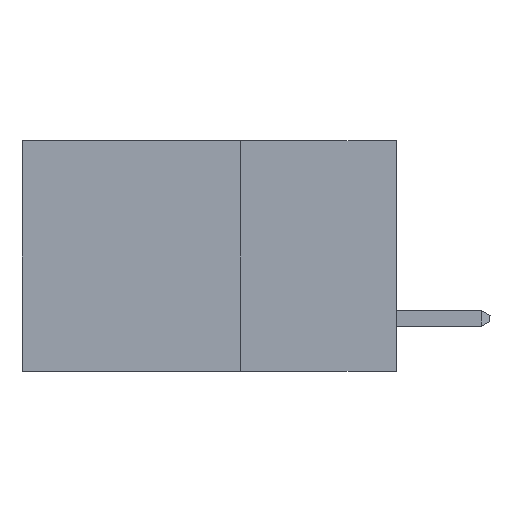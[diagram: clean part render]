
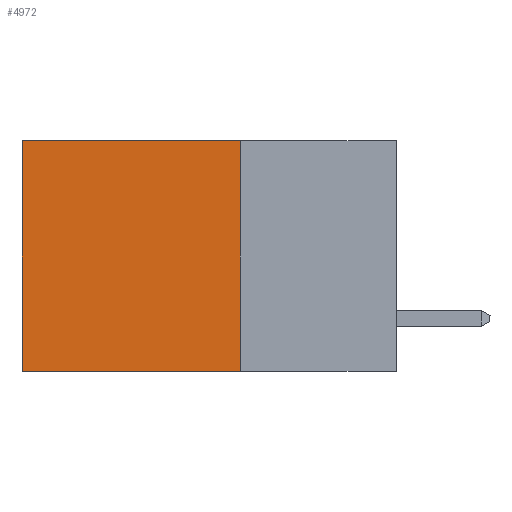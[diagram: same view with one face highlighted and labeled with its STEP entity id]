
A CAD part, left-side view. The second image highlights one B-rep face of the part: STEP entity #4972.
In plain terms, the highlighted planar face has unit normal (-1, 0, 0).
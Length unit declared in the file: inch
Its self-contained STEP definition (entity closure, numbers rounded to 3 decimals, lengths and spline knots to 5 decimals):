
#261 = EDGE_LOOP ( 'NONE', ( #2924, #5909, #6188, #5517 ) ) ;
#264 = LINE ( 'NONE', #614, #7894 ) ;
#614 = CARTESIAN_POINT ( 'NONE',  ( 0.2615, 0.25, -0.37 ) ) ;
#710 = CARTESIAN_POINT ( 'NONE',  ( 0.2615, 0.6, -0.37 ) ) ;
#723 = VERTEX_POINT ( 'NONE', #5499 ) ;
#1412 = DIRECTION ( 'NONE',  ( 0., 0., -1. ) ) ;
#1742 = LINE ( 'NONE', #710, #8904 ) ;
#1947 = VECTOR ( 'NONE', #8495, 39.37008 ) ;
#2290 = PLANE ( 'NONE',  #8635 ) ;
#2391 = VERTEX_POINT ( 'NONE', #5777 ) ;
#2392 = CARTESIAN_POINT ( 'NONE',  ( 0.2615, 0.25, -0.37 ) ) ;
#2921 = EDGE_CURVE ( 'NONE', #8026, #2391, #5956, .T. ) ;
#2924 = ORIENTED_EDGE ( 'NONE', *, *, #8230, .T. ) ;
#3650 = DIRECTION ( 'NONE',  ( 1., 0., 0. ) ) ;
#3850 = VECTOR ( 'NONE', #4699, 39.37008 ) ;
#3893 = CARTESIAN_POINT ( 'NONE',  ( 0.2615, 0.6, -0.37 ) ) ;
#4421 = DIRECTION ( 'NONE',  ( 0., 0., -1. ) ) ;
#4699 = DIRECTION ( 'NONE',  ( 0., 1., 0. ) ) ;
#4771 = FACE_OUTER_BOUND ( 'NONE', #261, .T. ) ;
#4972 = ADVANCED_FACE ( 'NONE', ( #4771 ), #2290, .F. ) ;
#5499 = CARTESIAN_POINT ( 'NONE',  ( 0.2615, 0.25, -0.37 ) ) ;
#5517 = ORIENTED_EDGE ( 'NONE', *, *, #2921, .T. ) ;
#5777 = CARTESIAN_POINT ( 'NONE',  ( 0.2615, 0.6, 0. ) ) ;
#5909 = ORIENTED_EDGE ( 'NONE', *, *, #6511, .F. ) ;
#5956 = LINE ( 'NONE', #8570, #1947 ) ;
#6188 = ORIENTED_EDGE ( 'NONE', *, *, #9245, .F. ) ;
#6511 = EDGE_CURVE ( 'NONE', #723, #7694, #8935, .T. ) ;
#7184 = CARTESIAN_POINT ( 'NONE',  ( 0.2615, 0.25, 0. ) ) ;
#7694 = VERTEX_POINT ( 'NONE', #3893 ) ;
#7894 = VECTOR ( 'NONE', #1412, 39.37008 ) ;
#8026 = VERTEX_POINT ( 'NONE', #7184 ) ;
#8230 = EDGE_CURVE ( 'NONE', #2391, #7694, #1742, .T. ) ;
#8495 = DIRECTION ( 'NONE',  ( 0., 1., 0. ) ) ;
#8570 = CARTESIAN_POINT ( 'NONE',  ( 0.2615, 0.25, 0. ) ) ;
#8635 = AXIS2_PLACEMENT_3D ( 'NONE', #9190, #3650, #4421 ) ;
#8904 = VECTOR ( 'NONE', #9233, 39.37008 ) ;
#8935 = LINE ( 'NONE', #2392, #3850 ) ;
#9190 = CARTESIAN_POINT ( 'NONE',  ( 0.2615, 0.25, -0.37 ) ) ;
#9233 = DIRECTION ( 'NONE',  ( 0., 0., -1. ) ) ;
#9245 = EDGE_CURVE ( 'NONE', #8026, #723, #264, .T. ) ;
